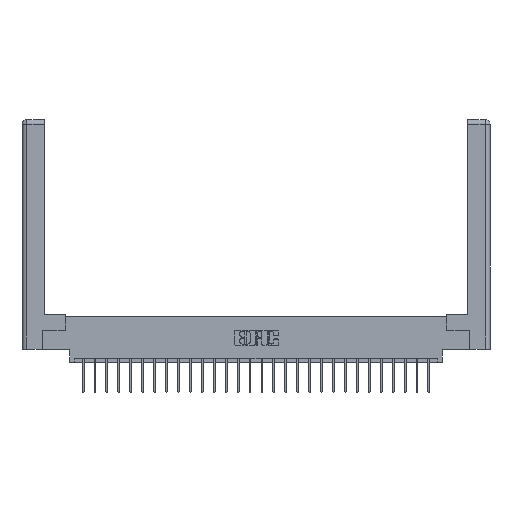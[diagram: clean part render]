
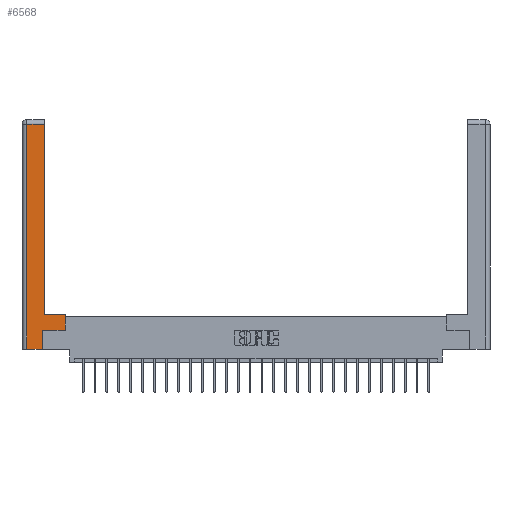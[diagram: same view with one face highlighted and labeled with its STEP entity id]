
A CAD part, top view. The second image highlights one B-rep face of the part: STEP entity #6568.
In plain terms, the highlighted planar face has unit normal (0, 0, 1).
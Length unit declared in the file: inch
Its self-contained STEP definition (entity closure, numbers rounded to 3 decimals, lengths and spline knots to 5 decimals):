
#264 = CARTESIAN_POINT ( 'NONE',  ( 0.295, 3., 0. ) ) ;
#1234 = LINE ( 'NONE', #12789, #13582 ) ;
#1807 = DIRECTION ( 'NONE',  ( 0., -1., 0. ) ) ;
#2181 = CARTESIAN_POINT ( 'NONE',  ( 0.295, 0.45, 0. ) ) ;
#2616 = CARTESIAN_POINT ( 'NONE',  ( 0.265, 0.245, 0. ) ) ;
#3045 = DIRECTION ( 'NONE',  ( 0., 1., 0. ) ) ;
#3048 = CARTESIAN_POINT ( 'NONE',  ( 0.295, 2.94, 0. ) ) ;
#3178 = PLANE ( 'NONE',  #5085 ) ;
#3694 = LINE ( 'NONE', #264, #20351 ) ;
#4012 = CARTESIAN_POINT ( 'NONE',  ( 0.565, 0.245, 0. ) ) ;
#5015 = ORIENTED_EDGE ( 'NONE', *, *, #22663, .T. ) ;
#5085 = AXIS2_PLACEMENT_3D ( 'NONE', #26469, #7615, #18172 ) ;
#5151 = EDGE_CURVE ( 'NONE', #11464, #17605, #17126, .T. ) ;
#5604 = VERTEX_POINT ( 'NONE', #10724 ) ;
#5835 = CARTESIAN_POINT ( 'NONE',  ( 0.295, 0.45, 0. ) ) ;
#6568 = ADVANCED_FACE ( 'NONE', ( #17057 ), #3178, .F. ) ;
#7615 = DIRECTION ( 'NONE',  ( 0., 0., -1. ) ) ;
#7900 = VERTEX_POINT ( 'NONE', #3048 ) ;
#10431 = CARTESIAN_POINT ( 'NONE',  ( 0.0615, 0., 0. ) ) ;
#10703 = EDGE_CURVE ( 'NONE', #13273, #5604, #27147, .T. ) ;
#10724 = CARTESIAN_POINT ( 'NONE',  ( 0.565, 0.45, 0. ) ) ;
#10951 = CARTESIAN_POINT ( 'NONE',  ( 0.0615, 0., 0. ) ) ;
#11464 = VERTEX_POINT ( 'NONE', #20308 ) ;
#11652 = VERTEX_POINT ( 'NONE', #15764 ) ;
#12789 = CARTESIAN_POINT ( 'NONE',  ( 0.0615, 2.94, 0. ) ) ;
#13273 = VERTEX_POINT ( 'NONE', #26054 ) ;
#13582 = VECTOR ( 'NONE', #23198, 39.37008 ) ;
#13644 = ORIENTED_EDGE ( 'NONE', *, *, #10703, .T. ) ;
#13665 = VERTEX_POINT ( 'NONE', #2616 ) ;
#14523 = EDGE_CURVE ( 'NONE', #5604, #25344, #27358, .T. ) ;
#14830 = EDGE_CURVE ( 'NONE', #25344, #7900, #3694, .T. ) ;
#15126 = DIRECTION ( 'NONE',  ( 0., 1., 0. ) ) ;
#15764 = CARTESIAN_POINT ( 'NONE',  ( 0.265, 0., 0. ) ) ;
#16061 = ORIENTED_EDGE ( 'NONE', *, *, #27286, .T. ) ;
#16209 = VECTOR ( 'NONE', #25748, 39.37008 ) ;
#16590 = DIRECTION ( 'NONE',  ( 0., 1., 0. ) ) ;
#16781 = EDGE_CURVE ( 'NONE', #13665, #13273, #24658, .T. ) ;
#17057 = FACE_OUTER_BOUND ( 'NONE', #20932, .T. ) ;
#17126 = LINE ( 'NONE', #10431, #26131 ) ;
#17605 = VERTEX_POINT ( 'NONE', #10951 ) ;
#18172 = DIRECTION ( 'NONE',  ( -1., 0., 0. ) ) ;
#18184 = LINE ( 'NONE', #27592, #16209 ) ;
#18315 = VECTOR ( 'NONE', #18909, 39.37008 ) ;
#18350 = ORIENTED_EDGE ( 'NONE', *, *, #16781, .T. ) ;
#18909 = DIRECTION ( 'NONE',  ( 1., 0., 0. ) ) ;
#19026 = ORIENTED_EDGE ( 'NONE', *, *, #14830, .T. ) ;
#19539 = ORIENTED_EDGE ( 'NONE', *, *, #14523, .T. ) ;
#19705 = VECTOR ( 'NONE', #22188, 39.37008 ) ;
#20308 = CARTESIAN_POINT ( 'NONE',  ( 0.0615, 2.94, 0. ) ) ;
#20351 = VECTOR ( 'NONE', #15126, 39.37008 ) ;
#20828 = VECTOR ( 'NONE', #3045, 39.37008 ) ;
#20932 = EDGE_LOOP ( 'NONE', ( #19026, #5015, #23449, #22204, #16061, #18350, #13644, #19539 ) ) ;
#21159 = LINE ( 'NONE', #23001, #22178 ) ;
#21970 = CARTESIAN_POINT ( 'NONE',  ( 0.565, 0.45, 0. ) ) ;
#22178 = VECTOR ( 'NONE', #16590, 39.37008 ) ;
#22188 = DIRECTION ( 'NONE',  ( -1., 0., 0. ) ) ;
#22204 = ORIENTED_EDGE ( 'NONE', *, *, #24328, .T. ) ;
#22663 = EDGE_CURVE ( 'NONE', #7900, #11464, #1234, .T. ) ;
#23001 = CARTESIAN_POINT ( 'NONE',  ( 0.265, 0.245, 0. ) ) ;
#23198 = DIRECTION ( 'NONE',  ( -1., 0., 0. ) ) ;
#23449 = ORIENTED_EDGE ( 'NONE', *, *, #5151, .T. ) ;
#24328 = EDGE_CURVE ( 'NONE', #17605, #11652, #18184, .T. ) ;
#24658 = LINE ( 'NONE', #4012, #18315 ) ;
#25344 = VERTEX_POINT ( 'NONE', #5835 ) ;
#25748 = DIRECTION ( 'NONE',  ( 1., 0., 0. ) ) ;
#26054 = CARTESIAN_POINT ( 'NONE',  ( 0.565, 0.245, 0. ) ) ;
#26131 = VECTOR ( 'NONE', #1807, 39.37008 ) ;
#26469 = CARTESIAN_POINT ( 'NONE',  ( 0., 0., 0. ) ) ;
#27147 = LINE ( 'NONE', #21970, #20828 ) ;
#27286 = EDGE_CURVE ( 'NONE', #11652, #13665, #21159, .T. ) ;
#27358 = LINE ( 'NONE', #2181, #19705 ) ;
#27592 = CARTESIAN_POINT ( 'NONE',  ( 0.265, 0., 0. ) ) ;
